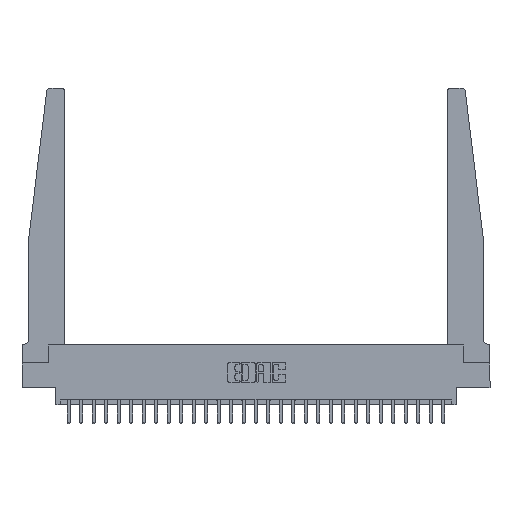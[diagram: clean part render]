
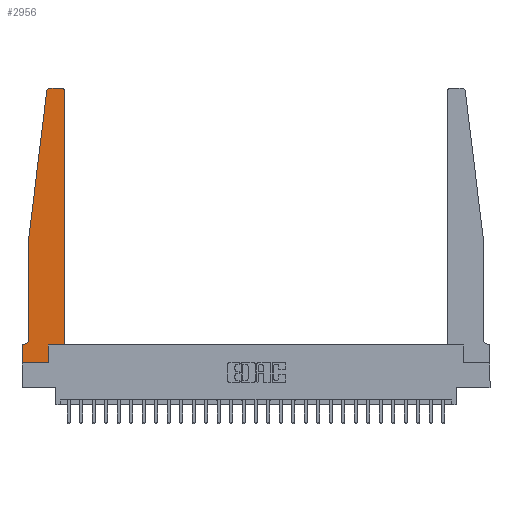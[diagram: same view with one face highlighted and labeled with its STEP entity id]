
A CAD part, top view. The second image highlights one B-rep face of the part: STEP entity #2956.
In plain terms, the highlighted planar face has unit normal (0, 0, 1).
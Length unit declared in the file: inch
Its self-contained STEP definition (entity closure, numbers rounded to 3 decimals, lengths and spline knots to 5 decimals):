
#344 = VECTOR ( 'NONE', #25892, 39.37008 ) ;
#1038 = CIRCLE ( 'NONE', #10590, 0.05 ) ;
#1210 = CARTESIAN_POINT ( 'NONE',  ( 0.065, 1.25, 0.37 ) ) ;
#1373 = CARTESIAN_POINT ( 'NONE',  ( 0.395, 2.75, 0.37 ) ) ;
#1414 = ORIENTED_EDGE ( 'NONE', *, *, #9658, .T. ) ;
#2529 = ORIENTED_EDGE ( 'NONE', *, *, #12286, .T. ) ;
#2634 = DIRECTION ( 'NONE',  ( -1., 0., 0. ) ) ;
#2667 = CARTESIAN_POINT ( 'NONE',  ( 0., 0., 0.37 ) ) ;
#2697 = VERTEX_POINT ( 'NONE', #15326 ) ;
#2731 = LINE ( 'NONE', #10689, #18083 ) ;
#2956 = ADVANCED_FACE ( 'NONE', ( #18981 ), #22304, .T. ) ;
#2960 = EDGE_LOOP ( 'NONE', ( #11481, #11789, #14512, #4767, #13850, #18285, #2529, #8341, #17460, #12820, #11593, #1414 ) ) ;
#2998 = AXIS2_PLACEMENT_3D ( 'NONE', #10905, #25259, #13012 ) ;
#3002 = VERTEX_POINT ( 'NONE', #26372 ) ;
#3017 = DIRECTION ( 'NONE',  ( 0., 0., 1. ) ) ;
#3389 = DIRECTION ( 'NONE',  ( -0.122, -0.992, 0. ) ) ;
#3639 = VERTEX_POINT ( 'NONE', #24374 ) ;
#4530 = CARTESIAN_POINT ( 'NONE',  ( 0.2605, 0.18, 0.37 ) ) ;
#4707 = CARTESIAN_POINT ( 'NONE',  ( 0.25, 2.75, 0.37 ) ) ;
#4767 = ORIENTED_EDGE ( 'NONE', *, *, #25336, .T. ) ;
#5251 = DIRECTION ( 'NONE',  ( 0., -1., 0. ) ) ;
#5630 = AXIS2_PLACEMENT_3D ( 'NONE', #15546, #3017, #17620 ) ;
#5740 = CARTESIAN_POINT ( 'NONE',  ( 0., 0.1875, 0.37 ) ) ;
#5967 = VECTOR ( 'NONE', #21109, 39.37008 ) ;
#5983 = CARTESIAN_POINT ( 'NONE',  ( 0., 0.1875, 0.37 ) ) ;
#6124 = CARTESIAN_POINT ( 'NONE',  ( 0.24675, 2.72367, 0.37 ) ) ;
#7244 = VERTEX_POINT ( 'NONE', #6124 ) ;
#7298 = VECTOR ( 'NONE', #24301, 39.37008 ) ;
#8153 = EDGE_CURVE ( 'NONE', #3002, #7244, #8836, .T. ) ;
#8341 = ORIENTED_EDGE ( 'NONE', *, *, #10827, .T. ) ;
#8836 = CIRCLE ( 'NONE', #5630, 0.03 ) ;
#9339 = DIRECTION ( 'NONE',  ( 0., 1., 0. ) ) ;
#9424 = CIRCLE ( 'NONE', #2998, 0.03 ) ;
#9658 = EDGE_CURVE ( 'NONE', #16935, #11733, #9424, .T. ) ;
#10010 = CARTESIAN_POINT ( 'NONE',  ( 0.2605, 0., 0.37 ) ) ;
#10213 = LINE ( 'NONE', #4530, #5967 ) ;
#10557 = EDGE_CURVE ( 'NONE', #19827, #16935, #10662, .T. ) ;
#10590 = AXIS2_PLACEMENT_3D ( 'NONE', #24605, #12342, #26570 ) ;
#10662 = LINE ( 'NONE', #19558, #26317 ) ;
#10689 = CARTESIAN_POINT ( 'NONE',  ( 0.065, 0.1875, 0.37 ) ) ;
#10827 = EDGE_CURVE ( 'NONE', #25535, #19101, #15883, .T. ) ;
#10905 = CARTESIAN_POINT ( 'NONE',  ( 0.395, 2.72, 0.37 ) ) ;
#10974 = VECTOR ( 'NONE', #25371, 39.37008 ) ;
#11179 = VERTEX_POINT ( 'NONE', #5983 ) ;
#11481 = ORIENTED_EDGE ( 'NONE', *, *, #13860, .T. ) ;
#11593 = ORIENTED_EDGE ( 'NONE', *, *, #10557, .T. ) ;
#11733 = VERTEX_POINT ( 'NONE', #1373 ) ;
#11789 = ORIENTED_EDGE ( 'NONE', *, *, #8153, .T. ) ;
#11846 = LINE ( 'NONE', #15665, #16717 ) ;
#11878 = CARTESIAN_POINT ( 'NONE',  ( 0.2605, 0.18, 0.37 ) ) ;
#12013 = CARTESIAN_POINT ( 'NONE',  ( 0.425, 0.18, 0.37 ) ) ;
#12037 = DIRECTION ( 'NONE',  ( 1., 0., 0. ) ) ;
#12286 = EDGE_CURVE ( 'NONE', #11179, #25535, #22519, .T. ) ;
#12342 = DIRECTION ( 'NONE',  ( 0., 0., -1. ) ) ;
#12802 = LINE ( 'NONE', #1210, #23096 ) ;
#12820 = ORIENTED_EDGE ( 'NONE', *, *, #25066, .T. ) ;
#12940 = VECTOR ( 'NONE', #2634, 39.37008 ) ;
#13012 = DIRECTION ( 'NONE',  ( 1., 0., 0. ) ) ;
#13705 = CARTESIAN_POINT ( 'NONE',  ( 0., 0., 0.37 ) ) ;
#13850 = ORIENTED_EDGE ( 'NONE', *, *, #23767, .T. ) ;
#13860 = EDGE_CURVE ( 'NONE', #11733, #3002, #24464, .T. ) ;
#14512 = ORIENTED_EDGE ( 'NONE', *, *, #16063, .T. ) ;
#14833 = CARTESIAN_POINT ( 'NONE',  ( 0.425, 0.18, 0.37 ) ) ;
#14896 = DIRECTION ( 'NONE',  ( -1., 0., 0. ) ) ;
#15326 = CARTESIAN_POINT ( 'NONE',  ( 0.065, 1.25, 0.37 ) ) ;
#15546 = CARTESIAN_POINT ( 'NONE',  ( 0.27653, 2.72, 0.37 ) ) ;
#15665 = CARTESIAN_POINT ( 'NONE',  ( 0.065, 1.25, 0.37 ) ) ;
#15724 = EDGE_CURVE ( 'NONE', #19101, #18353, #10213, .T. ) ;
#15883 = LINE ( 'NONE', #2667, #10974 ) ;
#16063 = EDGE_CURVE ( 'NONE', #7244, #2697, #12802, .T. ) ;
#16717 = VECTOR ( 'NONE', #5251, 39.37008 ) ;
#16935 = VERTEX_POINT ( 'NONE', #21131 ) ;
#17460 = ORIENTED_EDGE ( 'NONE', *, *, #15724, .T. ) ;
#17462 = VERTEX_POINT ( 'NONE', #23079 ) ;
#17620 = DIRECTION ( 'NONE',  ( 1., 0., 0. ) ) ;
#18083 = VECTOR ( 'NONE', #14896, 39.37008 ) ;
#18285 = ORIENTED_EDGE ( 'NONE', *, *, #23927, .T. ) ;
#18353 = VERTEX_POINT ( 'NONE', #11878 ) ;
#18981 = FACE_OUTER_BOUND ( 'NONE', #2960, .T. ) ;
#19101 = VERTEX_POINT ( 'NONE', #10010 ) ;
#19558 = CARTESIAN_POINT ( 'NONE',  ( 0.425, 0.18, 0.37 ) ) ;
#19809 = AXIS2_PLACEMENT_3D ( 'NONE', #5740, #24325, #12037 ) ;
#19827 = VERTEX_POINT ( 'NONE', #14833 ) ;
#21109 = DIRECTION ( 'NONE',  ( 0., 1., 0. ) ) ;
#21131 = CARTESIAN_POINT ( 'NONE',  ( 0.425, 2.72, 0.37 ) ) ;
#22304 = PLANE ( 'NONE',  #19809 ) ;
#22519 = LINE ( 'NONE', #13705, #344 ) ;
#23079 = CARTESIAN_POINT ( 'NONE',  ( 0.065, 0.2375, 0.37 ) ) ;
#23096 = VECTOR ( 'NONE', #3389, 39.37008 ) ;
#23126 = LINE ( 'NONE', #12013, #7298 ) ;
#23767 = EDGE_CURVE ( 'NONE', #17462, #3639, #1038, .T. ) ;
#23927 = EDGE_CURVE ( 'NONE', #3639, #11179, #2731, .T. ) ;
#24301 = DIRECTION ( 'NONE',  ( 1., 0., 0. ) ) ;
#24325 = DIRECTION ( 'NONE',  ( 0., 0., 1. ) ) ;
#24374 = CARTESIAN_POINT ( 'NONE',  ( 0.015, 0.1875, 0.37 ) ) ;
#24457 = CARTESIAN_POINT ( 'NONE',  ( 0., 0., 0.37 ) ) ;
#24464 = LINE ( 'NONE', #4707, #12940 ) ;
#24605 = CARTESIAN_POINT ( 'NONE',  ( 0.015, 0.2375, 0.37 ) ) ;
#25066 = EDGE_CURVE ( 'NONE', #18353, #19827, #23126, .T. ) ;
#25259 = DIRECTION ( 'NONE',  ( 0., 0., 1. ) ) ;
#25336 = EDGE_CURVE ( 'NONE', #2697, #17462, #11846, .T. ) ;
#25371 = DIRECTION ( 'NONE',  ( 1., 0., 0. ) ) ;
#25535 = VERTEX_POINT ( 'NONE', #24457 ) ;
#25892 = DIRECTION ( 'NONE',  ( 0., -1., 0. ) ) ;
#26317 = VECTOR ( 'NONE', #9339, 39.37008 ) ;
#26372 = CARTESIAN_POINT ( 'NONE',  ( 0.27653, 2.75, 0.37 ) ) ;
#26570 = DIRECTION ( 'NONE',  ( -1., 0., 0. ) ) ;
